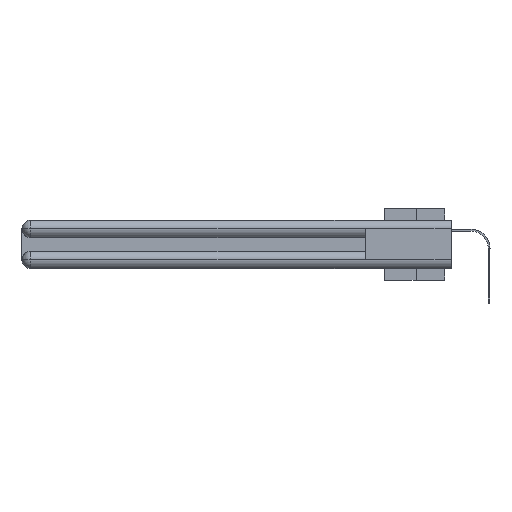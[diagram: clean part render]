
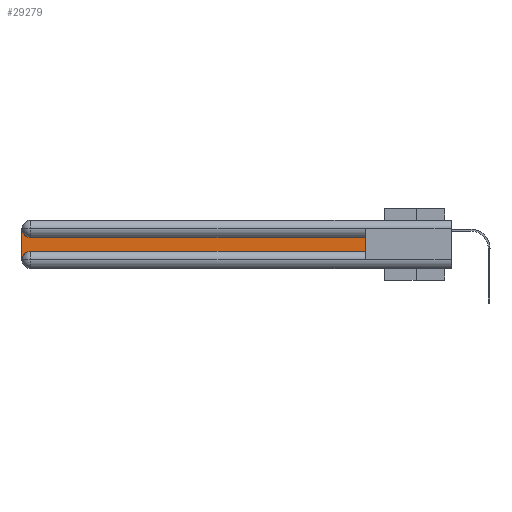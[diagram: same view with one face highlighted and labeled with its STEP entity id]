
A CAD part, left-side view. The second image highlights one B-rep face of the part: STEP entity #29279.
In plain terms, the highlighted planar face has unit normal (-1, 0, 0).
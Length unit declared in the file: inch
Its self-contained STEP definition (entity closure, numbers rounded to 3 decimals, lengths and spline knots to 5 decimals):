
#48 = VERTEX_POINT ( 'NONE', #681 ) ;
#681 = CARTESIAN_POINT ( 'NONE',  ( 0.075, 0.6, -0.2175 ) ) ;
#1365 = FACE_OUTER_BOUND ( 'NONE', #18868, .T. ) ;
#2643 = ORIENTED_EDGE ( 'NONE', *, *, #11768, .T. ) ;
#3889 = DIRECTION ( 'NONE',  ( 0., 0., -1. ) ) ;
#4552 = EDGE_CURVE ( 'NONE', #48, #35868, #30222, .T. ) ;
#4921 = DIRECTION ( 'NONE',  ( 0., -1., 0. ) ) ;
#5590 = ORIENTED_EDGE ( 'NONE', *, *, #36497, .T. ) ;
#6447 = ORIENTED_EDGE ( 'NONE', *, *, #29320, .T. ) ;
#7917 = VERTEX_POINT ( 'NONE', #30133 ) ;
#10332 = CARTESIAN_POINT ( 'NONE',  ( 0.075, 3., -0.2775 ) ) ;
#10382 = CARTESIAN_POINT ( 'NONE',  ( 0.075, 3., -0.0625 ) ) ;
#10820 = CARTESIAN_POINT ( 'NONE',  ( 0.075, 0.6, -0.2175 ) ) ;
#11115 = VERTEX_POINT ( 'NONE', #30125 ) ;
#11768 = EDGE_CURVE ( 'NONE', #27318, #16338, #31404, .T. ) ;
#12257 = ORIENTED_EDGE ( 'NONE', *, *, #35100, .T. ) ;
#14256 = CARTESIAN_POINT ( 'NONE',  ( 0.075, 3., -0.2175 ) ) ;
#15230 = ORIENTED_EDGE ( 'NONE', *, *, #35859, .T. ) ;
#15872 = DIRECTION ( 'NONE',  ( 1., 0., 0. ) ) ;
#16126 = LINE ( 'NONE', #27420, #27115 ) ;
#16338 = VERTEX_POINT ( 'NONE', #10332 ) ;
#16773 = CARTESIAN_POINT ( 'NONE',  ( 0.075, 0.6, -0.2175 ) ) ;
#16959 = VECTOR ( 'NONE', #4921, 39.37008 ) ;
#17762 = AXIS2_PLACEMENT_3D ( 'NONE', #32837, #24521, #27527 ) ;
#18767 = DIRECTION ( 'NONE',  ( 0., 1., 0. ) ) ;
#18868 = EDGE_LOOP ( 'NONE', ( #15230, #6447, #2643, #5590, #12257, #30987 ) ) ;
#19617 = AXIS2_PLACEMENT_3D ( 'NONE', #27153, #15872, #21899 ) ;
#19962 = AXIS2_PLACEMENT_3D ( 'NONE', #21388, #21002, #3889 ) ;
#21002 = DIRECTION ( 'NONE',  ( 1., 0., 0. ) ) ;
#21388 = CARTESIAN_POINT ( 'NONE',  ( 0.075, 2.94, -0.2775 ) ) ;
#21899 = DIRECTION ( 'NONE',  ( 0., 0., -1. ) ) ;
#22143 = CARTESIAN_POINT ( 'NONE',  ( 0.075, 0.6, -0.1225 ) ) ;
#22317 = VECTOR ( 'NONE', #28378, 39.37008 ) ;
#24521 = DIRECTION ( 'NONE',  ( 1., 0., 0. ) ) ;
#24766 = CIRCLE ( 'NONE', #19962, 0.06 ) ;
#27115 = VECTOR ( 'NONE', #18767, 39.37008 ) ;
#27153 = CARTESIAN_POINT ( 'NONE',  ( 0.075, 2.94, -0.0625 ) ) ;
#27318 = VERTEX_POINT ( 'NONE', #10382 ) ;
#27420 = CARTESIAN_POINT ( 'NONE',  ( 0.075, 0.6, -0.1225 ) ) ;
#27527 = DIRECTION ( 'NONE',  ( 0., 0., -1. ) ) ;
#28074 = LINE ( 'NONE', #16773, #16959 ) ;
#28378 = DIRECTION ( 'NONE',  ( 0., 0., -1. ) ) ;
#29002 = VECTOR ( 'NONE', #30784, 39.37008 ) ;
#29279 = ADVANCED_FACE ( 'NONE', ( #1365 ), #36253, .F. ) ;
#29320 = EDGE_CURVE ( 'NONE', #7917, #27318, #30406, .T. ) ;
#30125 = CARTESIAN_POINT ( 'NONE',  ( 0.075, 2.94, -0.2175 ) ) ;
#30133 = CARTESIAN_POINT ( 'NONE',  ( 0.075, 2.94, -0.1225 ) ) ;
#30222 = LINE ( 'NONE', #10820, #29002 ) ;
#30406 = CIRCLE ( 'NONE', #19617, 0.06 ) ;
#30784 = DIRECTION ( 'NONE',  ( 0., 0., 1. ) ) ;
#30987 = ORIENTED_EDGE ( 'NONE', *, *, #4552, .T. ) ;
#31404 = LINE ( 'NONE', #14256, #22317 ) ;
#32837 = CARTESIAN_POINT ( 'NONE',  ( 0.075, 3., -0.1225 ) ) ;
#35100 = EDGE_CURVE ( 'NONE', #11115, #48, #28074, .T. ) ;
#35859 = EDGE_CURVE ( 'NONE', #35868, #7917, #16126, .T. ) ;
#35868 = VERTEX_POINT ( 'NONE', #22143 ) ;
#36253 = PLANE ( 'NONE',  #17762 ) ;
#36497 = EDGE_CURVE ( 'NONE', #16338, #11115, #24766, .T. ) ;
